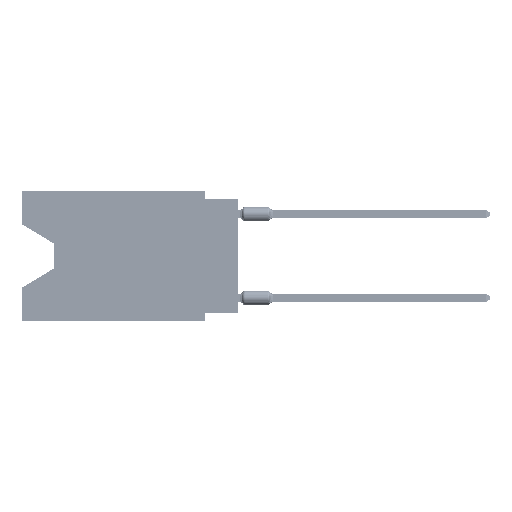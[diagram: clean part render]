
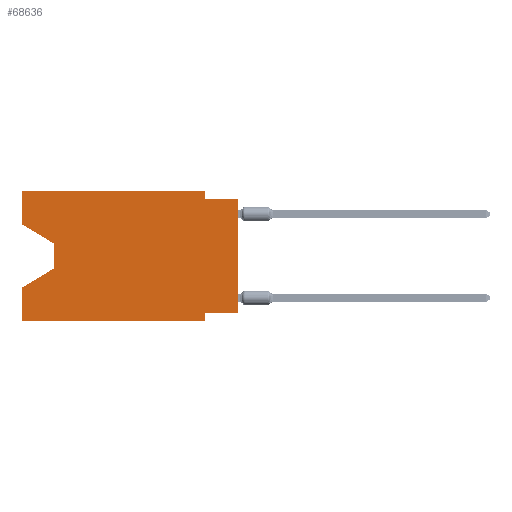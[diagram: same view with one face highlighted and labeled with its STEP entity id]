
A CAD part, left-side view. The second image highlights one B-rep face of the part: STEP entity #68636.
In plain terms, the highlighted planar face has unit normal (-1, 0, 0).
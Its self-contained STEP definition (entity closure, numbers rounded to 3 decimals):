
#284 = VECTOR ( 'NONE', #70206, 1000. ) ;
#800 = VECTOR ( 'NONE', #4223, 1000. ) ;
#2263 = CARTESIAN_POINT ( 'NONE',  ( 0., 2.54, -9.906 ) ) ;
#3457 = DIRECTION ( 'NONE',  ( 0., -1., 0. ) ) ;
#3780 = ORIENTED_EDGE ( 'NONE', *, *, #14003, .F. ) ;
#4223 = DIRECTION ( 'NONE',  ( 0., 0., -1. ) ) ;
#4985 = LINE ( 'NONE', #37080, #11569 ) ;
#5134 = FACE_OUTER_BOUND ( 'NONE', #16240, .T. ) ;
#6514 = VECTOR ( 'NONE', #33106, 1000. ) ;
#7130 = VERTEX_POINT ( 'NONE', #11643 ) ;
#8262 = EDGE_CURVE ( 'NONE', #7130, #16831, #28574, .T. ) ;
#9180 = CARTESIAN_POINT ( 'NONE',  ( 0., 16.383, 0. ) ) ;
#9353 = VECTOR ( 'NONE', #51319, 1000. ) ;
#10560 = CARTESIAN_POINT ( 'NONE',  ( 0., 0., 0. ) ) ;
#11542 = VECTOR ( 'NONE', #71233, 1000. ) ;
#11569 = VECTOR ( 'NONE', #65658, 1000. ) ;
#11643 = CARTESIAN_POINT ( 'NONE',  ( 0., 13.97, -5.893 ) ) ;
#12767 = VERTEX_POINT ( 'NONE', #2263 ) ;
#13299 = ORIENTED_EDGE ( 'NONE', *, *, #35311, .F. ) ;
#14003 = EDGE_CURVE ( 'NONE', #16298, #12767, #70493, .T. ) ;
#14235 = CARTESIAN_POINT ( 'NONE',  ( 0., 2.54, 0. ) ) ;
#16240 = EDGE_LOOP ( 'NONE', ( #47455, #49720, #70740, #13299, #42212, #3780, #64272, #20874, #27163, #60145, #32387, #64828 ) ) ;
#16298 = VERTEX_POINT ( 'NONE', #73792 ) ;
#16478 = CARTESIAN_POINT ( 'NONE',  ( 0., 2.54, -9.906 ) ) ;
#16831 = VERTEX_POINT ( 'NONE', #32591 ) ;
#18072 = CARTESIAN_POINT ( 'NONE',  ( 0., 16.383, 0. ) ) ;
#19083 = EDGE_CURVE ( 'NONE', #29976, #22214, #58836, .T. ) ;
#19515 = DIRECTION ( 'NONE',  ( 0., 1., 0. ) ) ;
#20874 = ORIENTED_EDGE ( 'NONE', *, *, #66241, .T. ) ;
#22214 = VERTEX_POINT ( 'NONE', #66413 ) ;
#22296 = CARTESIAN_POINT ( 'NONE',  ( 0., 13.97, -4.013 ) ) ;
#22628 = VERTEX_POINT ( 'NONE', #14235 ) ;
#23503 = DIRECTION ( 'NONE',  ( 0., 0., -1. ) ) ;
#24862 = EDGE_CURVE ( 'NONE', #70793, #7130, #34037, .T. ) ;
#25378 = VECTOR ( 'NONE', #23503, 1000. ) ;
#27163 = ORIENTED_EDGE ( 'NONE', *, *, #19083, .F. ) ;
#28574 = LINE ( 'NONE', #69264, #39801 ) ;
#29090 = EDGE_CURVE ( 'NONE', #57283, #12767, #4985, .T. ) ;
#29976 = VERTEX_POINT ( 'NONE', #63998 ) ;
#29997 = EDGE_CURVE ( 'NONE', #35405, #40794, #57753, .T. ) ;
#30383 = EDGE_CURVE ( 'NONE', #22628, #29976, #52074, .T. ) ;
#32387 = ORIENTED_EDGE ( 'NONE', *, *, #75992, .F. ) ;
#32591 = CARTESIAN_POINT ( 'NONE',  ( 0., 16.383, -7.36 ) ) ;
#33106 = DIRECTION ( 'NONE',  ( 0., 0., 1. ) ) ;
#34037 = LINE ( 'NONE', #22296, #800 ) ;
#35311 = EDGE_CURVE ( 'NONE', #57283, #16831, #65813, .T. ) ;
#35405 = VERTEX_POINT ( 'NONE', #76834 ) ;
#36081 = DIRECTION ( 'NONE',  ( 0., 0., -1. ) ) ;
#37080 = CARTESIAN_POINT ( 'NONE',  ( 0., 16.383, -9.906 ) ) ;
#37109 = CARTESIAN_POINT ( 'NONE',  ( 0., 0., -9.271 ) ) ;
#39801 = VECTOR ( 'NONE', #63762, 1000. ) ;
#40794 = VERTEX_POINT ( 'NONE', #57009 ) ;
#41195 = DIRECTION ( 'NONE',  ( 1., 0., 0. ) ) ;
#41210 = VECTOR ( 'NONE', #47750, 1000. ) ;
#42212 = ORIENTED_EDGE ( 'NONE', *, *, #29090, .T. ) ;
#43778 = CARTESIAN_POINT ( 'NONE',  ( 0., 16.383, -9.906 ) ) ;
#46237 = LINE ( 'NONE', #10560, #9353 ) ;
#47455 = ORIENTED_EDGE ( 'NONE', *, *, #53131, .T. ) ;
#47750 = DIRECTION ( 'NONE',  ( 0., 0., -1. ) ) ;
#49720 = ORIENTED_EDGE ( 'NONE', *, *, #24862, .T. ) ;
#50874 = CARTESIAN_POINT ( 'NONE',  ( 0., 16.383, 0. ) ) ;
#51319 = DIRECTION ( 'NONE',  ( 0., 0., 1. ) ) ;
#52074 = LINE ( 'NONE', #63818, #25378 ) ;
#53131 = EDGE_CURVE ( 'NONE', #35405, #70793, #54371, .T. ) ;
#54300 = CARTESIAN_POINT ( 'NONE',  ( 0., 13.97, -4.013 ) ) ;
#54371 = LINE ( 'NONE', #59115, #11542 ) ;
#54583 = VECTOR ( 'NONE', #19515, 1000. ) ;
#54603 = VERTEX_POINT ( 'NONE', #64487 ) ;
#54638 = AXIS2_PLACEMENT_3D ( 'NONE', #18072, #41195, #36081 ) ;
#57009 = CARTESIAN_POINT ( 'NONE',  ( 0., 16.383, 0. ) ) ;
#57283 = VERTEX_POINT ( 'NONE', #43778 ) ;
#57530 = LINE ( 'NONE', #50874, #77380 ) ;
#57753 = LINE ( 'NONE', #9180, #6514 ) ;
#58836 = LINE ( 'NONE', #69425, #284 ) ;
#59115 = CARTESIAN_POINT ( 'NONE',  ( 0., 16.383, -2.546 ) ) ;
#60145 = ORIENTED_EDGE ( 'NONE', *, *, #30383, .F. ) ;
#60231 = LINE ( 'NONE', #37109, #54583 ) ;
#63762 = DIRECTION ( 'NONE',  ( 0., 0.855, -0.519 ) ) ;
#63818 = CARTESIAN_POINT ( 'NONE',  ( 0., 2.54, 0. ) ) ;
#63998 = CARTESIAN_POINT ( 'NONE',  ( 0., 2.54, -0.635 ) ) ;
#64272 = ORIENTED_EDGE ( 'NONE', *, *, #68010, .F. ) ;
#64487 = CARTESIAN_POINT ( 'NONE',  ( 0., 0., -9.271 ) ) ;
#64828 = ORIENTED_EDGE ( 'NONE', *, *, #29997, .F. ) ;
#65441 = CARTESIAN_POINT ( 'NONE',  ( 0., 16.383, 0. ) ) ;
#65658 = DIRECTION ( 'NONE',  ( 0., -1., 0. ) ) ;
#65813 = LINE ( 'NONE', #65441, #76079 ) ;
#66241 = EDGE_CURVE ( 'NONE', #54603, #22214, #46237, .T. ) ;
#66413 = CARTESIAN_POINT ( 'NONE',  ( 0., 0., -0.635 ) ) ;
#68010 = EDGE_CURVE ( 'NONE', #54603, #16298, #60231, .T. ) ;
#68636 = ADVANCED_FACE ( 'NONE', ( #5134 ), #76831, .F. ) ;
#69264 = CARTESIAN_POINT ( 'NONE',  ( 0., 13.97, -5.893 ) ) ;
#69425 = CARTESIAN_POINT ( 'NONE',  ( 0., 0., -0.635 ) ) ;
#70206 = DIRECTION ( 'NONE',  ( 0., -1., 0. ) ) ;
#70493 = LINE ( 'NONE', #16478, #41210 ) ;
#70565 = DIRECTION ( 'NONE',  ( 0., 0., 1. ) ) ;
#70740 = ORIENTED_EDGE ( 'NONE', *, *, #8262, .T. ) ;
#70793 = VERTEX_POINT ( 'NONE', #54300 ) ;
#71233 = DIRECTION ( 'NONE',  ( 0., -0.855, -0.519 ) ) ;
#73792 = CARTESIAN_POINT ( 'NONE',  ( 0., 2.54, -9.271 ) ) ;
#75992 = EDGE_CURVE ( 'NONE', #40794, #22628, #57530, .T. ) ;
#76079 = VECTOR ( 'NONE', #70565, 1000. ) ;
#76831 = PLANE ( 'NONE',  #54638 ) ;
#76834 = CARTESIAN_POINT ( 'NONE',  ( 0., 16.383, -2.546 ) ) ;
#77380 = VECTOR ( 'NONE', #3457, 1000. ) ;
